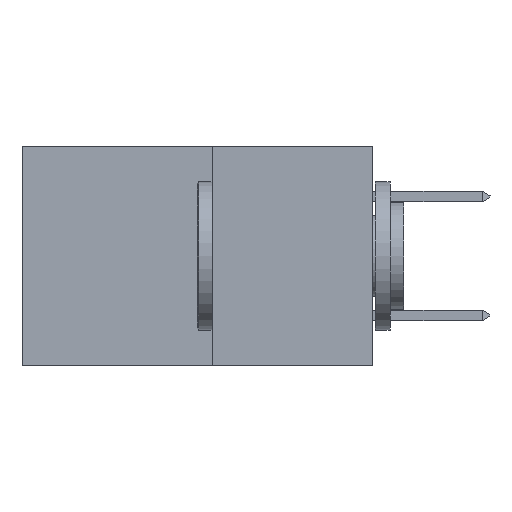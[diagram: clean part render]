
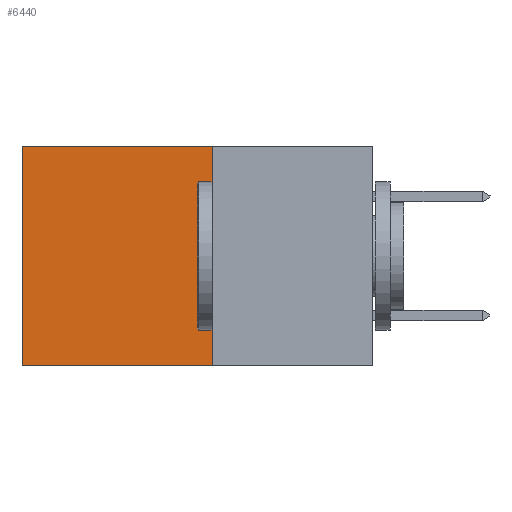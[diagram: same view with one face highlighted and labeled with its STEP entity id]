
A CAD part, left-side view. The second image highlights one B-rep face of the part: STEP entity #6440.
In plain terms, the highlighted planar face has unit normal (-1, 0, 0).
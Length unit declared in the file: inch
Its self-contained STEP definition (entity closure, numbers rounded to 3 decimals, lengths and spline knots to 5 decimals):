
#210 = CARTESIAN_POINT ( 'NONE',  ( 0.277, 0.27, 0. ) ) ;
#401 = VECTOR ( 'NONE', #7848, 39.37008 ) ;
#407 = VERTEX_POINT ( 'NONE', #1562 ) ;
#411 = CARTESIAN_POINT ( 'NONE',  ( 0.277, 0.27, -0.37 ) ) ;
#1077 = LINE ( 'NONE', #1537, #6431 ) ;
#1102 = PLANE ( 'NONE',  #1898 ) ;
#1244 = EDGE_LOOP ( 'NONE', ( #6357, #4836, #1443, #3282 ) ) ;
#1443 = ORIENTED_EDGE ( 'NONE', *, *, #6339, .F. ) ;
#1537 = CARTESIAN_POINT ( 'NONE',  ( 0.277, 0.27, 0. ) ) ;
#1562 = CARTESIAN_POINT ( 'NONE',  ( 0.277, 0.59, 0. ) ) ;
#1683 = DIRECTION ( 'NONE',  ( 0., 0., -1. ) ) ;
#1812 = EDGE_CURVE ( 'NONE', #407, #6569, #5594, .T. ) ;
#1815 = LINE ( 'NONE', #7123, #5388 ) ;
#1898 = AXIS2_PLACEMENT_3D ( 'NONE', #411, #6483, #2491 ) ;
#1958 = CARTESIAN_POINT ( 'NONE',  ( 0.277, 0.59, -0.37 ) ) ;
#2179 = CARTESIAN_POINT ( 'NONE',  ( 0.277, 0.59, -0.37 ) ) ;
#2228 = DIRECTION ( 'NONE',  ( 0., 1., 0. ) ) ;
#2376 = CARTESIAN_POINT ( 'NONE',  ( 0.277, 0.27, -0.37 ) ) ;
#2491 = DIRECTION ( 'NONE',  ( 0., 0., -1. ) ) ;
#3222 = DIRECTION ( 'NONE',  ( 0., 1., 0. ) ) ;
#3282 = ORIENTED_EDGE ( 'NONE', *, *, #6178, .T. ) ;
#3286 = CARTESIAN_POINT ( 'NONE',  ( 0.277, 0.27, -0.37 ) ) ;
#4123 = VERTEX_POINT ( 'NONE', #3286 ) ;
#4836 = ORIENTED_EDGE ( 'NONE', *, *, #7097, .F. ) ;
#4994 = LINE ( 'NONE', #2376, #8162 ) ;
#5388 = VECTOR ( 'NONE', #3222, 39.37008 ) ;
#5594 = LINE ( 'NONE', #2179, #401 ) ;
#6178 = EDGE_CURVE ( 'NONE', #7421, #407, #1077, .T. ) ;
#6339 = EDGE_CURVE ( 'NONE', #7421, #4123, #4994, .T. ) ;
#6357 = ORIENTED_EDGE ( 'NONE', *, *, #1812, .T. ) ;
#6431 = VECTOR ( 'NONE', #2228, 39.37008 ) ;
#6440 = ADVANCED_FACE ( 'NONE', ( #7794 ), #1102, .F. ) ;
#6483 = DIRECTION ( 'NONE',  ( 1., 0., 0. ) ) ;
#6569 = VERTEX_POINT ( 'NONE', #1958 ) ;
#7097 = EDGE_CURVE ( 'NONE', #4123, #6569, #1815, .T. ) ;
#7123 = CARTESIAN_POINT ( 'NONE',  ( 0.277, 0.27, -0.37 ) ) ;
#7421 = VERTEX_POINT ( 'NONE', #210 ) ;
#7794 = FACE_OUTER_BOUND ( 'NONE', #1244, .T. ) ;
#7848 = DIRECTION ( 'NONE',  ( 0., 0., -1. ) ) ;
#8162 = VECTOR ( 'NONE', #1683, 39.37008 ) ;
